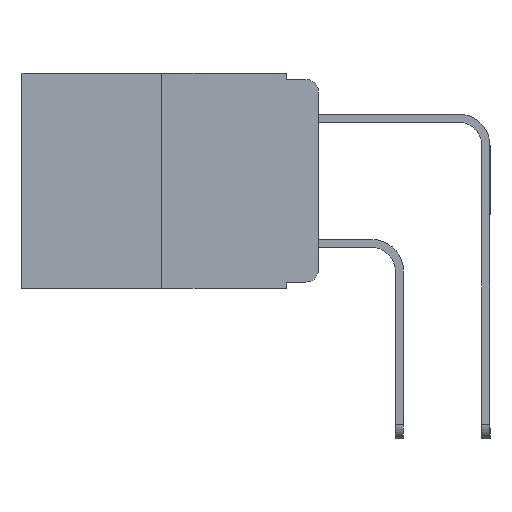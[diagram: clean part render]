
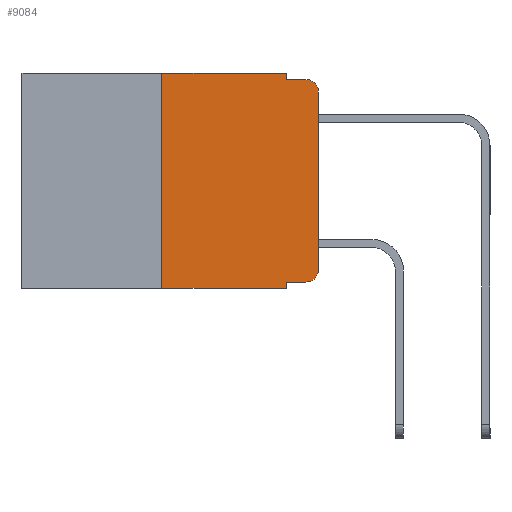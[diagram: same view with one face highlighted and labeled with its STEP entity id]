
A CAD part, left-side view. The second image highlights one B-rep face of the part: STEP entity #9084.
In plain terms, the highlighted planar face has unit normal (-1, 0, 0).
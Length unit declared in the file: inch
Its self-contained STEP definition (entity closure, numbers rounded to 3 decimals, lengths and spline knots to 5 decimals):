
#64 = VERTEX_POINT ( 'NONE', #7978 ) ;
#120 = CARTESIAN_POINT ( 'NONE',  ( 0., 0.051, -0.343 ) ) ;
#495 = PLANE ( 'NONE',  #2025 ) ;
#636 = ORIENTED_EDGE ( 'NONE', *, *, #1137, .F. ) ;
#857 = EDGE_CURVE ( 'NONE', #1617, #879, #1047, .T. ) ;
#869 = LINE ( 'NONE', #11517, #6312 ) ;
#879 = VERTEX_POINT ( 'NONE', #3477 ) ;
#886 = AXIS2_PLACEMENT_3D ( 'NONE', #3563, #3909, #6483 ) ;
#920 = ORIENTED_EDGE ( 'NONE', *, *, #12974, .T. ) ;
#979 = ORIENTED_EDGE ( 'NONE', *, *, #2635, .F. ) ;
#1047 = LINE ( 'NONE', #3698, #9244 ) ;
#1137 = EDGE_CURVE ( 'NONE', #8369, #64, #869, .T. ) ;
#1147 = CARTESIAN_POINT ( 'NONE',  ( 0., 0., -0.313 ) ) ;
#1493 = VERTEX_POINT ( 'NONE', #1147 ) ;
#1617 = VERTEX_POINT ( 'NONE', #9730 ) ;
#1622 = CARTESIAN_POINT ( 'NONE',  ( 0., 0.473, 0. ) ) ;
#1700 = DIRECTION ( 'NONE',  ( 0., -1., 0. ) ) ;
#1931 = VECTOR ( 'NONE', #12443, 39.37008 ) ;
#2011 = CARTESIAN_POINT ( 'NONE',  ( 0., 0.051, 0. ) ) ;
#2012 = ORIENTED_EDGE ( 'NONE', *, *, #4826, .F. ) ;
#2025 = AXIS2_PLACEMENT_3D ( 'NONE', #1622, #2735, #10052 ) ;
#2412 = VECTOR ( 'NONE', #1700, 39.37008 ) ;
#2538 = VERTEX_POINT ( 'NONE', #10470 ) ;
#2635 = EDGE_CURVE ( 'NONE', #2538, #12268, #12157, .T. ) ;
#2735 = DIRECTION ( 'NONE',  ( 1., 0., 0. ) ) ;
#3477 = CARTESIAN_POINT ( 'NONE',  ( 0., 0.02, -0.01 ) ) ;
#3563 = CARTESIAN_POINT ( 'NONE',  ( 0., 0.02, -0.03 ) ) ;
#3698 = CARTESIAN_POINT ( 'NONE',  ( 0., 0.051, -0.01 ) ) ;
#3761 = DIRECTION ( 'NONE',  ( 0., 0., 1. ) ) ;
#3785 = LINE ( 'NONE', #12767, #11943 ) ;
#3801 = VERTEX_POINT ( 'NONE', #6789 ) ;
#3831 = CARTESIAN_POINT ( 'NONE',  ( 0., 0.051, 0. ) ) ;
#3909 = DIRECTION ( 'NONE',  ( -1., 0., 0. ) ) ;
#3945 = CARTESIAN_POINT ( 'NONE',  ( 0., 0.473, -0.343 ) ) ;
#4789 = VECTOR ( 'NONE', #6736, 39.37008 ) ;
#4826 = EDGE_CURVE ( 'NONE', #5752, #1617, #7503, .T. ) ;
#5058 = EDGE_CURVE ( 'NONE', #2538, #6112, #7841, .T. ) ;
#5210 = AXIS2_PLACEMENT_3D ( 'NONE', #6344, #13345, #7413 ) ;
#5533 = EDGE_CURVE ( 'NONE', #3801, #879, #10179, .T. ) ;
#5618 = CARTESIAN_POINT ( 'NONE',  ( 0., 0.051, 0. ) ) ;
#5723 = ORIENTED_EDGE ( 'NONE', *, *, #5058, .T. ) ;
#5752 = VERTEX_POINT ( 'NONE', #2011 ) ;
#5789 = EDGE_CURVE ( 'NONE', #64, #5752, #10316, .T. ) ;
#5820 = ORIENTED_EDGE ( 'NONE', *, *, #5533, .T. ) ;
#6112 = VERTEX_POINT ( 'NONE', #8994 ) ;
#6312 = VECTOR ( 'NONE', #3761, 39.37008 ) ;
#6344 = CARTESIAN_POINT ( 'NONE',  ( 0., 0.02, -0.313 ) ) ;
#6396 = CARTESIAN_POINT ( 'NONE',  ( 0., 0.473, 0. ) ) ;
#6451 = EDGE_CURVE ( 'NONE', #6112, #1493, #7147, .T. ) ;
#6483 = DIRECTION ( 'NONE',  ( 0., 0., -1. ) ) ;
#6736 = DIRECTION ( 'NONE',  ( 0., 0., -1. ) ) ;
#6756 = DIRECTION ( 'NONE',  ( 0., 0., 1. ) ) ;
#6789 = CARTESIAN_POINT ( 'NONE',  ( 0., 0., -0.03 ) ) ;
#6811 = ORIENTED_EDGE ( 'NONE', *, *, #5789, .F. ) ;
#6835 = CARTESIAN_POINT ( 'NONE',  ( 0., 0.051, -0.333 ) ) ;
#7147 = CIRCLE ( 'NONE', #5210, 0.02 ) ;
#7161 = DIRECTION ( 'NONE',  ( 0., 0., -1. ) ) ;
#7413 = DIRECTION ( 'NONE',  ( 0., 0., -1. ) ) ;
#7503 = LINE ( 'NONE', #3831, #12488 ) ;
#7778 = DIRECTION ( 'NONE',  ( 0., -1., 0. ) ) ;
#7841 = LINE ( 'NONE', #6835, #10190 ) ;
#7864 = ORIENTED_EDGE ( 'NONE', *, *, #857, .F. ) ;
#7978 = CARTESIAN_POINT ( 'NONE',  ( 0., 0.25, 0. ) ) ;
#8109 = LINE ( 'NONE', #3945, #2412 ) ;
#8369 = VERTEX_POINT ( 'NONE', #12140 ) ;
#8565 = DIRECTION ( 'NONE',  ( 0., -1., 0. ) ) ;
#8994 = CARTESIAN_POINT ( 'NONE',  ( 0., 0.02, -0.333 ) ) ;
#9084 = ADVANCED_FACE ( 'NONE', ( #12548 ), #495, .F. ) ;
#9155 = ORIENTED_EDGE ( 'NONE', *, *, #6451, .T. ) ;
#9228 = EDGE_LOOP ( 'NONE', ( #920, #5820, #7864, #2012, #6811, #636, #11309, #979, #5723, #9155 ) ) ;
#9244 = VECTOR ( 'NONE', #8565, 39.37008 ) ;
#9730 = CARTESIAN_POINT ( 'NONE',  ( 0., 0.051, -0.01 ) ) ;
#10052 = DIRECTION ( 'NONE',  ( 0., 0., -1. ) ) ;
#10179 = CIRCLE ( 'NONE', #886, 0.02 ) ;
#10190 = VECTOR ( 'NONE', #7778, 39.37008 ) ;
#10316 = LINE ( 'NONE', #6396, #1931 ) ;
#10470 = CARTESIAN_POINT ( 'NONE',  ( 0., 0.051, -0.333 ) ) ;
#11309 = ORIENTED_EDGE ( 'NONE', *, *, #11709, .T. ) ;
#11517 = CARTESIAN_POINT ( 'NONE',  ( 0., 0.25, 0. ) ) ;
#11709 = EDGE_CURVE ( 'NONE', #8369, #12268, #8109, .T. ) ;
#11943 = VECTOR ( 'NONE', #6756, 39.37008 ) ;
#12140 = CARTESIAN_POINT ( 'NONE',  ( 0., 0.25, -0.343 ) ) ;
#12157 = LINE ( 'NONE', #5618, #4789 ) ;
#12268 = VERTEX_POINT ( 'NONE', #120 ) ;
#12443 = DIRECTION ( 'NONE',  ( 0., -1., 0. ) ) ;
#12488 = VECTOR ( 'NONE', #7161, 39.37008 ) ;
#12548 = FACE_OUTER_BOUND ( 'NONE', #9228, .T. ) ;
#12767 = CARTESIAN_POINT ( 'NONE',  ( 0., 0., 0. ) ) ;
#12974 = EDGE_CURVE ( 'NONE', #1493, #3801, #3785, .T. ) ;
#13345 = DIRECTION ( 'NONE',  ( -1., 0., 0. ) ) ;
